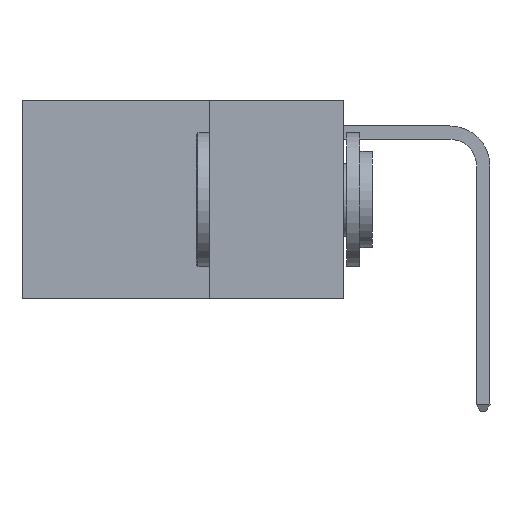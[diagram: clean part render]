
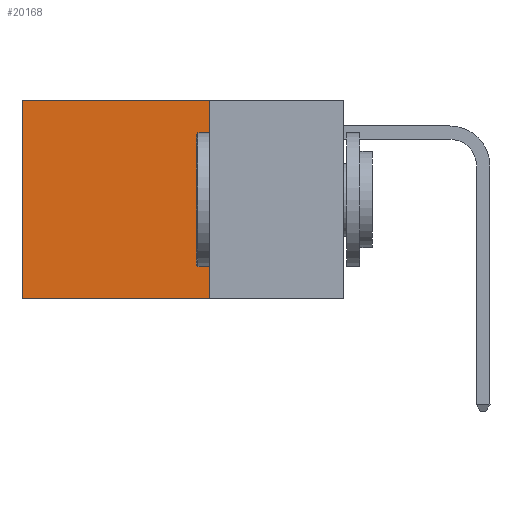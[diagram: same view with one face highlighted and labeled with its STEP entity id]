
A CAD part, left-side view. The second image highlights one B-rep face of the part: STEP entity #20168.
In plain terms, the highlighted planar face has unit normal (-1, 0, 0).
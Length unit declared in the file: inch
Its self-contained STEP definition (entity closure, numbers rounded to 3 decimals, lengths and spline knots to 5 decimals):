
#222 = CARTESIAN_POINT ( 'NONE',  ( 0.2625, 0.25, 0. ) ) ;
#861 = EDGE_CURVE ( 'NONE', #4585, #2015, #15839, .T. ) ;
#1113 = EDGE_CURVE ( 'NONE', #8203, #11488, #3452, .T. ) ;
#1173 = CARTESIAN_POINT ( 'NONE',  ( 0.2625, 0.25, 0. ) ) ;
#1521 = AXIS2_PLACEMENT_3D ( 'NONE', #10104, #18668, #12070 ) ;
#1732 = DIRECTION ( 'NONE',  ( 0., 1., 0. ) ) ;
#2015 = VERTEX_POINT ( 'NONE', #11522 ) ;
#2282 = CARTESIAN_POINT ( 'NONE',  ( 0.2625, 0.6, -0.37 ) ) ;
#2392 = VECTOR ( 'NONE', #4627, 39.37008 ) ;
#2907 = LINE ( 'NONE', #12866, #6387 ) ;
#3452 = LINE ( 'NONE', #19919, #7209 ) ;
#3678 = EDGE_CURVE ( 'NONE', #4585, #8203, #9048, .T. ) ;
#4585 = VERTEX_POINT ( 'NONE', #222 ) ;
#4627 = DIRECTION ( 'NONE',  ( 0., 0., -1. ) ) ;
#4646 = DIRECTION ( 'NONE',  ( 0., 0., -1. ) ) ;
#5166 = ORIENTED_EDGE ( 'NONE', *, *, #3678, .F. ) ;
#5769 = EDGE_LOOP ( 'NONE', ( #8329, #17995, #5166, #14490 ) ) ;
#6387 = VECTOR ( 'NONE', #4646, 39.37008 ) ;
#7209 = VECTOR ( 'NONE', #1732, 39.37008 ) ;
#7625 = CARTESIAN_POINT ( 'NONE',  ( 0.2625, 0.25, 0. ) ) ;
#8203 = VERTEX_POINT ( 'NONE', #19137 ) ;
#8329 = ORIENTED_EDGE ( 'NONE', *, *, #10517, .T. ) ;
#8693 = PLANE ( 'NONE',  #1521 ) ;
#9048 = LINE ( 'NONE', #1173, #2392 ) ;
#10104 = CARTESIAN_POINT ( 'NONE',  ( 0.2625, 0.25, 0. ) ) ;
#10517 = EDGE_CURVE ( 'NONE', #2015, #11488, #2907, .T. ) ;
#11488 = VERTEX_POINT ( 'NONE', #2282 ) ;
#11522 = CARTESIAN_POINT ( 'NONE',  ( 0.2625, 0.6, 0. ) ) ;
#12070 = DIRECTION ( 'NONE',  ( 0., 0., -1. ) ) ;
#12866 = CARTESIAN_POINT ( 'NONE',  ( 0.2625, 0.6, 0. ) ) ;
#14490 = ORIENTED_EDGE ( 'NONE', *, *, #861, .T. ) ;
#15839 = LINE ( 'NONE', #7625, #18569 ) ;
#17995 = ORIENTED_EDGE ( 'NONE', *, *, #1113, .F. ) ;
#18569 = VECTOR ( 'NONE', #19225, 39.37008 ) ;
#18668 = DIRECTION ( 'NONE',  ( 1., 0., 0. ) ) ;
#19137 = CARTESIAN_POINT ( 'NONE',  ( 0.2625, 0.25, -0.37 ) ) ;
#19225 = DIRECTION ( 'NONE',  ( 0., 1., 0. ) ) ;
#19667 = FACE_OUTER_BOUND ( 'NONE', #5769, .T. ) ;
#19919 = CARTESIAN_POINT ( 'NONE',  ( 0.2625, 0.25, -0.37 ) ) ;
#20168 = ADVANCED_FACE ( 'NONE', ( #19667 ), #8693, .F. ) ;
